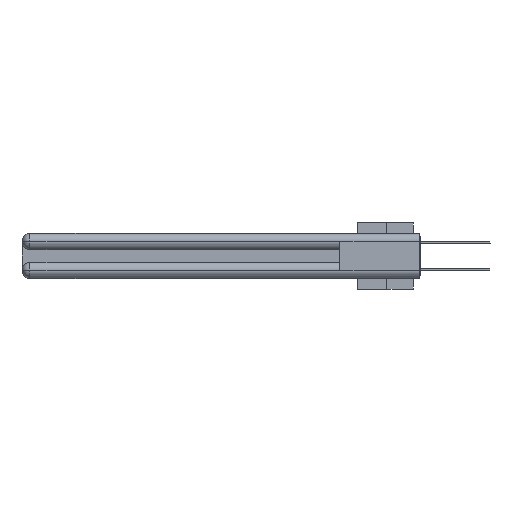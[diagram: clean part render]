
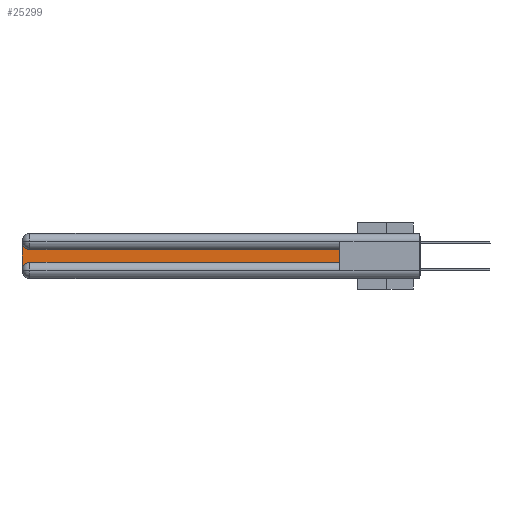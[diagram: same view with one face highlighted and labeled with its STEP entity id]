
A CAD part, left-side view. The second image highlights one B-rep face of the part: STEP entity #25299.
In plain terms, the highlighted planar face has unit normal (-1, 0, 0).
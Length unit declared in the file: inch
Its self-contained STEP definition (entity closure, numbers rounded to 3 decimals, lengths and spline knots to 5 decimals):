
#1215 = DIRECTION ( 'NONE',  ( 0., 0., -1. ) ) ;
#1285 = AXIS2_PLACEMENT_3D ( 'NONE', #25138, #28118, #25271 ) ;
#1464 = LINE ( 'NONE', #32696, #31150 ) ;
#1830 = ORIENTED_EDGE ( 'NONE', *, *, #29796, .T. ) ;
#2005 = CARTESIAN_POINT ( 'NONE',  ( 0.075, 0.6, -0.2175 ) ) ;
#2155 = CARTESIAN_POINT ( 'NONE',  ( 0.075, 3., -0.1225 ) ) ;
#4350 = EDGE_CURVE ( 'NONE', #28476, #36083, #1464, .T. ) ;
#6216 = EDGE_CURVE ( 'NONE', #17493, #28476, #31021, .T. ) ;
#6416 = CARTESIAN_POINT ( 'NONE',  ( 0.075, 0.6, -0.1225 ) ) ;
#7470 = CARTESIAN_POINT ( 'NONE',  ( 0.075, 3., -0.2775 ) ) ;
#7496 = CARTESIAN_POINT ( 'NONE',  ( 0.075, 2.94, -0.2175 ) ) ;
#7610 = DIRECTION ( 'NONE',  ( 0., 0., -1. ) ) ;
#7741 = PLANE ( 'NONE',  #35547 ) ;
#7904 = ORIENTED_EDGE ( 'NONE', *, *, #19543, .T. ) ;
#7975 = DIRECTION ( 'NONE',  ( 0., -1., 0. ) ) ;
#8017 = EDGE_CURVE ( 'NONE', #12505, #17493, #30393, .T. ) ;
#8137 = DIRECTION ( 'NONE',  ( 1., 0., 0. ) ) ;
#8383 = ORIENTED_EDGE ( 'NONE', *, *, #4350, .T. ) ;
#8913 = ORIENTED_EDGE ( 'NONE', *, *, #34476, .T. ) ;
#10700 = CARTESIAN_POINT ( 'NONE',  ( 0.075, 0.6, -0.2175 ) ) ;
#10946 = CARTESIAN_POINT ( 'NONE',  ( 0.075, 0.6, -0.1225 ) ) ;
#11298 = VERTEX_POINT ( 'NONE', #13289 ) ;
#11580 = VECTOR ( 'NONE', #7975, 39.37008 ) ;
#12505 = VERTEX_POINT ( 'NONE', #7470 ) ;
#12796 = CARTESIAN_POINT ( 'NONE',  ( 0.075, 2.94, -0.0625 ) ) ;
#13289 = CARTESIAN_POINT ( 'NONE',  ( 0.075, 2.94, -0.1225 ) ) ;
#14928 = DIRECTION ( 'NONE',  ( 0., 0., 1. ) ) ;
#15129 = AXIS2_PLACEMENT_3D ( 'NONE', #12796, #33658, #1215 ) ;
#17215 = ORIENTED_EDGE ( 'NONE', *, *, #6216, .T. ) ;
#17493 = VERTEX_POINT ( 'NONE', #7496 ) ;
#18016 = CIRCLE ( 'NONE', #15129, 0.06 ) ;
#18192 = ORIENTED_EDGE ( 'NONE', *, *, #8017, .T. ) ;
#19050 = VERTEX_POINT ( 'NONE', #32387 ) ;
#19267 = EDGE_LOOP ( 'NONE', ( #7904, #8913, #1830, #18192, #17215, #8383 ) ) ;
#19543 = EDGE_CURVE ( 'NONE', #36083, #11298, #32194, .T. ) ;
#22338 = DIRECTION ( 'NONE',  ( 0., 0., -1. ) ) ;
#22953 = DIRECTION ( 'NONE',  ( 0., 1., 0. ) ) ;
#25138 = CARTESIAN_POINT ( 'NONE',  ( 0.075, 2.94, -0.2775 ) ) ;
#25271 = DIRECTION ( 'NONE',  ( 0., 0., -1. ) ) ;
#25299 = ADVANCED_FACE ( 'NONE', ( #30651 ), #7741, .F. ) ;
#27980 = VECTOR ( 'NONE', #22953, 39.37008 ) ;
#28118 = DIRECTION ( 'NONE',  ( 1., 0., 0. ) ) ;
#28476 = VERTEX_POINT ( 'NONE', #10700 ) ;
#29139 = CARTESIAN_POINT ( 'NONE',  ( 0.075, 3., -0.2175 ) ) ;
#29796 = EDGE_CURVE ( 'NONE', #19050, #12505, #32417, .T. ) ;
#30393 = CIRCLE ( 'NONE', #1285, 0.06 ) ;
#30651 = FACE_OUTER_BOUND ( 'NONE', #19267, .T. ) ;
#31021 = LINE ( 'NONE', #2005, #11580 ) ;
#31150 = VECTOR ( 'NONE', #14928, 39.37008 ) ;
#32194 = LINE ( 'NONE', #10946, #27980 ) ;
#32387 = CARTESIAN_POINT ( 'NONE',  ( 0.075, 3., -0.0625 ) ) ;
#32417 = LINE ( 'NONE', #29139, #36096 ) ;
#32696 = CARTESIAN_POINT ( 'NONE',  ( 0.075, 0.6, -0.2175 ) ) ;
#33658 = DIRECTION ( 'NONE',  ( 1., 0., 0. ) ) ;
#34476 = EDGE_CURVE ( 'NONE', #11298, #19050, #18016, .T. ) ;
#35547 = AXIS2_PLACEMENT_3D ( 'NONE', #2155, #8137, #7610 ) ;
#36083 = VERTEX_POINT ( 'NONE', #6416 ) ;
#36096 = VECTOR ( 'NONE', #22338, 39.37008 ) ;
